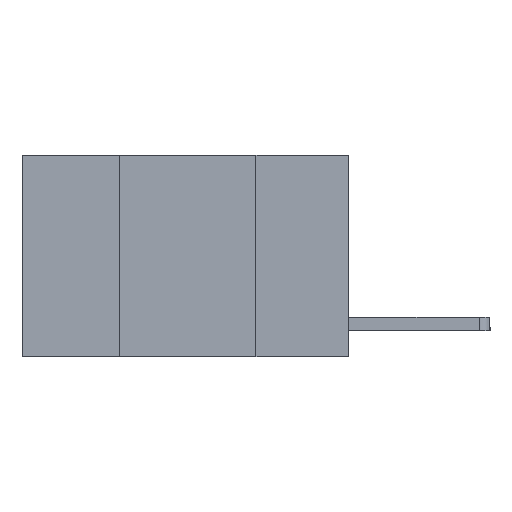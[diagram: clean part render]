
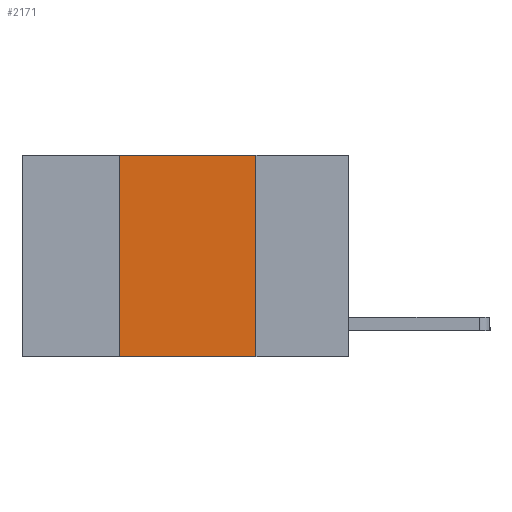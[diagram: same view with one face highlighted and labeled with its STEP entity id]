
A CAD part, left-side view. The second image highlights one B-rep face of the part: STEP entity #2171.
In plain terms, the highlighted planar face has unit normal (-1, 0, 0).
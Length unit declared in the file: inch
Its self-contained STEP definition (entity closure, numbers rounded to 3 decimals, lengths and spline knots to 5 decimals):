
#374 = PLANE ( 'NONE',  #8445 ) ;
#969 = VECTOR ( 'NONE', #9144, 39.37008 ) ;
#1074 = ORIENTED_EDGE ( 'NONE', *, *, #6129, .T. ) ;
#1155 = CARTESIAN_POINT ( 'NONE',  ( 0., 0.17, 0. ) ) ;
#1184 = VERTEX_POINT ( 'NONE', #6750 ) ;
#1609 = CARTESIAN_POINT ( 'NONE',  ( 0., 0.6, -0.37 ) ) ;
#1765 = LINE ( 'NONE', #5614, #10060 ) ;
#1999 = CARTESIAN_POINT ( 'NONE',  ( 0., 0.42, 0. ) ) ;
#2171 = ADVANCED_FACE ( 'NONE', ( #3587 ), #374, .F. ) ;
#2254 = ORIENTED_EDGE ( 'NONE', *, *, #3284, .F. ) ;
#2599 = CARTESIAN_POINT ( 'NONE',  ( 0., 0.42, -0.37 ) ) ;
#2984 = ORIENTED_EDGE ( 'NONE', *, *, #7478, .F. ) ;
#3284 = EDGE_CURVE ( 'NONE', #8004, #4026, #8880, .T. ) ;
#3587 = FACE_OUTER_BOUND ( 'NONE', #3628, .T. ) ;
#3625 = LINE ( 'NONE', #1999, #4822 ) ;
#3628 = EDGE_LOOP ( 'NONE', ( #2254, #2984, #8422, #1074 ) ) ;
#4026 = VERTEX_POINT ( 'NONE', #9278 ) ;
#4181 = VERTEX_POINT ( 'NONE', #2599 ) ;
#4278 = DIRECTION ( 'NONE',  ( 0., 0., 1. ) ) ;
#4384 = CARTESIAN_POINT ( 'NONE',  ( 0., 0.17, 0. ) ) ;
#4551 = LINE ( 'NONE', #1609, #969 ) ;
#4822 = VECTOR ( 'NONE', #4278, 39.37008 ) ;
#4854 = VECTOR ( 'NONE', #8118, 39.37008 ) ;
#5614 = CARTESIAN_POINT ( 'NONE',  ( 0., 0.6, 0. ) ) ;
#5856 = DIRECTION ( 'NONE',  ( 1., 0., 0. ) ) ;
#6129 = EDGE_CURVE ( 'NONE', #4181, #4026, #4551, .T. ) ;
#6750 = CARTESIAN_POINT ( 'NONE',  ( 0., 0.42, 0. ) ) ;
#7396 = CARTESIAN_POINT ( 'NONE',  ( 0., 0.6, 0. ) ) ;
#7478 = EDGE_CURVE ( 'NONE', #1184, #8004, #1765, .T. ) ;
#7960 = EDGE_CURVE ( 'NONE', #4181, #1184, #3625, .T. ) ;
#8004 = VERTEX_POINT ( 'NONE', #4384 ) ;
#8118 = DIRECTION ( 'NONE',  ( 0., 0., -1. ) ) ;
#8314 = DIRECTION ( 'NONE',  ( 0., 0., -1. ) ) ;
#8422 = ORIENTED_EDGE ( 'NONE', *, *, #7960, .F. ) ;
#8445 = AXIS2_PLACEMENT_3D ( 'NONE', #7396, #5856, #8314 ) ;
#8880 = LINE ( 'NONE', #1155, #4854 ) ;
#9144 = DIRECTION ( 'NONE',  ( 0., -1., 0. ) ) ;
#9278 = CARTESIAN_POINT ( 'NONE',  ( 0., 0.17, -0.37 ) ) ;
#9512 = DIRECTION ( 'NONE',  ( 0., -1., 0. ) ) ;
#10060 = VECTOR ( 'NONE', #9512, 39.37008 ) ;
